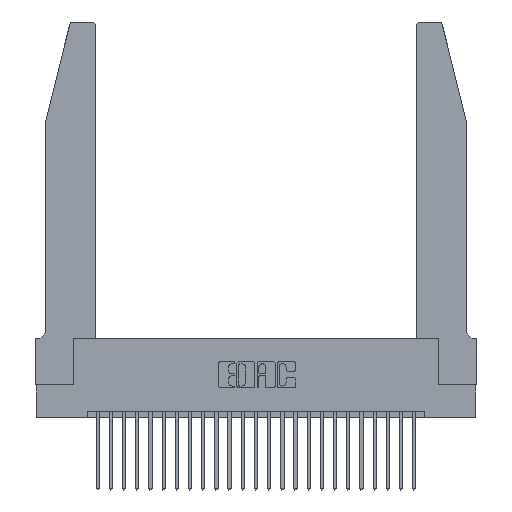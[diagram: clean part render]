
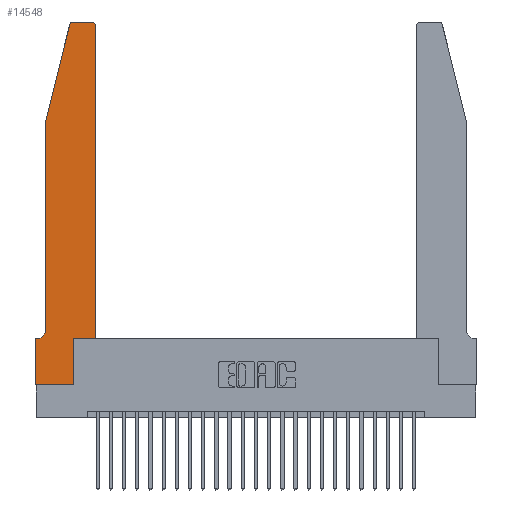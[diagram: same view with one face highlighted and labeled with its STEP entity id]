
A CAD part, top view. The second image highlights one B-rep face of the part: STEP entity #14548.
In plain terms, the highlighted planar face has unit normal (0, 0, 1).
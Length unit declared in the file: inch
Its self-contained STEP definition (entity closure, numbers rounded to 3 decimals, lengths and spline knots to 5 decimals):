
#36 = VERTEX_POINT ( 'NONE', #14016 ) ;
#263 = DIRECTION ( 'NONE',  ( 0., 0., 1. ) ) ;
#291 = LINE ( 'NONE', #5372, #10953 ) ;
#344 = EDGE_CURVE ( 'NONE', #24148, #15300, #1412, .T. ) ;
#492 = ORIENTED_EDGE ( 'NONE', *, *, #16540, .T. ) ;
#658 = ORIENTED_EDGE ( 'NONE', *, *, #19632, .T. ) ;
#778 = EDGE_CURVE ( 'NONE', #15684, #18872, #24986, .T. ) ;
#1412 = LINE ( 'NONE', #10094, #22748 ) ;
#1613 = VERTEX_POINT ( 'NONE', #23605 ) ;
#1673 = CARTESIAN_POINT ( 'NONE',  ( 0.2605, 2.75, 0.37 ) ) ;
#1739 = CARTESIAN_POINT ( 'NONE',  ( 0., 0., 0.37 ) ) ;
#2112 = DIRECTION ( 'NONE',  ( 1., 0., 0. ) ) ;
#2191 = LINE ( 'NONE', #9698, #5884 ) ;
#2285 = DIRECTION ( 'NONE',  ( -0.239, -0.971, 0. ) ) ;
#2352 = CIRCLE ( 'NONE', #20772, 0.03 ) ;
#2535 = DIRECTION ( 'NONE',  ( -1., 0., 0. ) ) ;
#2890 = EDGE_CURVE ( 'NONE', #19598, #7865, #18308, .T. ) ;
#2990 = EDGE_CURVE ( 'NONE', #1613, #24148, #15118, .T. ) ;
#3523 = DIRECTION ( 'NONE',  ( 0., -1., 0. ) ) ;
#4007 = ORIENTED_EDGE ( 'NONE', *, *, #13706, .T. ) ;
#4213 = CARTESIAN_POINT ( 'NONE',  ( 0.284, 2.75, 0.37 ) ) ;
#4340 = CARTESIAN_POINT ( 'NONE',  ( 0.0755, 0.42, 0.37 ) ) ;
#5181 = LINE ( 'NONE', #7431, #25022 ) ;
#5372 = CARTESIAN_POINT ( 'NONE',  ( 0.0755, 2., 0.37 ) ) ;
#5884 = VECTOR ( 'NONE', #13817, 39.37008 ) ;
#6173 = DIRECTION ( 'NONE',  ( 1., 0., 0. ) ) ;
#6222 = VERTEX_POINT ( 'NONE', #17054 ) ;
#6780 = VECTOR ( 'NONE', #10260, 39.37008 ) ;
#7431 = CARTESIAN_POINT ( 'NONE',  ( 0.4505, 0.35, 0.37 ) ) ;
#7589 = LINE ( 'NONE', #14651, #11856 ) ;
#7645 = DIRECTION ( 'NONE',  ( 1., 0., 0. ) ) ;
#7865 = VERTEX_POINT ( 'NONE', #21898 ) ;
#8156 = VERTEX_POINT ( 'NONE', #22649 ) ;
#8384 = ORIENTED_EDGE ( 'NONE', *, *, #26680, .T. ) ;
#8492 = CIRCLE ( 'NONE', #15035, 0.07 ) ;
#8553 = EDGE_CURVE ( 'NONE', #17662, #8156, #2191, .T. ) ;
#9293 = FACE_OUTER_BOUND ( 'NONE', #12403, .T. ) ;
#9482 = EDGE_CURVE ( 'NONE', #14634, #6222, #8492, .T. ) ;
#9528 = ORIENTED_EDGE ( 'NONE', *, *, #778, .T. ) ;
#9671 = VECTOR ( 'NONE', #3523, 39.37008 ) ;
#9698 = CARTESIAN_POINT ( 'NONE',  ( 0.4505, 0.35, 0.37 ) ) ;
#9895 = CARTESIAN_POINT ( 'NONE',  ( 0.4205, 2.75, 0.37 ) ) ;
#10076 = CARTESIAN_POINT ( 'NONE',  ( 0., 0., 0.37 ) ) ;
#10094 = CARTESIAN_POINT ( 'NONE',  ( 0., 0., 0.37 ) ) ;
#10260 = DIRECTION ( 'NONE',  ( -1., 0., 0. ) ) ;
#10777 = CARTESIAN_POINT ( 'NONE',  ( 0.2865, 0.35, 0.37 ) ) ;
#10888 = EDGE_CURVE ( 'NONE', #6222, #1613, #12367, .T. ) ;
#10953 = VECTOR ( 'NONE', #17778, 39.37008 ) ;
#11238 = CARTESIAN_POINT ( 'NONE',  ( 0.0055, 0.42, 0.37 ) ) ;
#11336 = ORIENTED_EDGE ( 'NONE', *, *, #22390, .T. ) ;
#11856 = VECTOR ( 'NONE', #26687, 39.37008 ) ;
#11934 = ORIENTED_EDGE ( 'NONE', *, *, #2890, .T. ) ;
#12044 = ORIENTED_EDGE ( 'NONE', *, *, #344, .T. ) ;
#12268 = VECTOR ( 'NONE', #2285, 39.37008 ) ;
#12367 = LINE ( 'NONE', #18373, #6780 ) ;
#12403 = EDGE_LOOP ( 'NONE', ( #9528, #658, #11934, #4007, #14754, #22758, #18171, #12044, #11336, #17003, #8384, #492 ) ) ;
#12950 = CARTESIAN_POINT ( 'NONE',  ( 0.284, 2.72, 0.37 ) ) ;
#13081 = AXIS2_PLACEMENT_3D ( 'NONE', #26704, #14672, #2112 ) ;
#13283 = DIRECTION ( 'NONE',  ( -1., 0., 0. ) ) ;
#13701 = DIRECTION ( 'NONE',  ( 0., 1., 0. ) ) ;
#13706 = EDGE_CURVE ( 'NONE', #7865, #14634, #291, .T. ) ;
#13817 = DIRECTION ( 'NONE',  ( 1., 0., 0. ) ) ;
#14016 = CARTESIAN_POINT ( 'NONE',  ( 0.4505, 2.72, 0.37 ) ) ;
#14548 = ADVANCED_FACE ( 'NONE', ( #9293 ), #22471, .T. ) ;
#14634 = VERTEX_POINT ( 'NONE', #4340 ) ;
#14651 = CARTESIAN_POINT ( 'NONE',  ( 0.2865, 0.35, 0.37 ) ) ;
#14672 = DIRECTION ( 'NONE',  ( 0., 0., 1. ) ) ;
#14754 = ORIENTED_EDGE ( 'NONE', *, *, #9482, .T. ) ;
#14992 = DIRECTION ( 'NONE',  ( 1., 0., 0. ) ) ;
#15035 = AXIS2_PLACEMENT_3D ( 'NONE', #11238, #25373, #13283 ) ;
#15118 = LINE ( 'NONE', #1739, #9671 ) ;
#15300 = VERTEX_POINT ( 'NONE', #18838 ) ;
#15684 = VERTEX_POINT ( 'NONE', #9895 ) ;
#16540 = EDGE_CURVE ( 'NONE', #36, #15684, #22221, .T. ) ;
#16861 = CARTESIAN_POINT ( 'NONE',  ( 0.25487, 2.72718, 0.37 ) ) ;
#17003 = ORIENTED_EDGE ( 'NONE', *, *, #8553, .T. ) ;
#17054 = CARTESIAN_POINT ( 'NONE',  ( 0.0055, 0.35, 0.37 ) ) ;
#17662 = VERTEX_POINT ( 'NONE', #10777 ) ;
#17778 = DIRECTION ( 'NONE',  ( 0., -1., 0. ) ) ;
#18171 = ORIENTED_EDGE ( 'NONE', *, *, #2990, .T. ) ;
#18308 = LINE ( 'NONE', #19961, #12268 ) ;
#18373 = CARTESIAN_POINT ( 'NONE',  ( 0.0755, 0.35, 0.37 ) ) ;
#18544 = DIRECTION ( 'NONE',  ( 0., 0., 1. ) ) ;
#18838 = CARTESIAN_POINT ( 'NONE',  ( 0.2865, 0., 0.37 ) ) ;
#18872 = VERTEX_POINT ( 'NONE', #4213 ) ;
#19598 = VERTEX_POINT ( 'NONE', #16861 ) ;
#19632 = EDGE_CURVE ( 'NONE', #18872, #19598, #2352, .T. ) ;
#19961 = CARTESIAN_POINT ( 'NONE',  ( 0.0755, 2., 0.37 ) ) ;
#20205 = AXIS2_PLACEMENT_3D ( 'NONE', #26486, #18544, #6173 ) ;
#20772 = AXIS2_PLACEMENT_3D ( 'NONE', #12950, #263, #14992 ) ;
#21898 = CARTESIAN_POINT ( 'NONE',  ( 0.0755, 2., 0.37 ) ) ;
#22221 = CIRCLE ( 'NONE', #13081, 0.03 ) ;
#22390 = EDGE_CURVE ( 'NONE', #15300, #17662, #7589, .T. ) ;
#22471 = PLANE ( 'NONE',  #20205 ) ;
#22649 = CARTESIAN_POINT ( 'NONE',  ( 0.4505, 0.35, 0.37 ) ) ;
#22748 = VECTOR ( 'NONE', #7645, 39.37008 ) ;
#22758 = ORIENTED_EDGE ( 'NONE', *, *, #10888, .T. ) ;
#23605 = CARTESIAN_POINT ( 'NONE',  ( 0., 0.35, 0.37 ) ) ;
#24148 = VERTEX_POINT ( 'NONE', #10076 ) ;
#24354 = VECTOR ( 'NONE', #2535, 39.37008 ) ;
#24986 = LINE ( 'NONE', #1673, #24354 ) ;
#25022 = VECTOR ( 'NONE', #13701, 39.37008 ) ;
#25373 = DIRECTION ( 'NONE',  ( 0., 0., -1. ) ) ;
#26486 = CARTESIAN_POINT ( 'NONE',  ( 0., 0.35, 0.37 ) ) ;
#26680 = EDGE_CURVE ( 'NONE', #8156, #36, #5181, .T. ) ;
#26687 = DIRECTION ( 'NONE',  ( 0., 1., 0. ) ) ;
#26704 = CARTESIAN_POINT ( 'NONE',  ( 0.4205, 2.72, 0.37 ) ) ;
